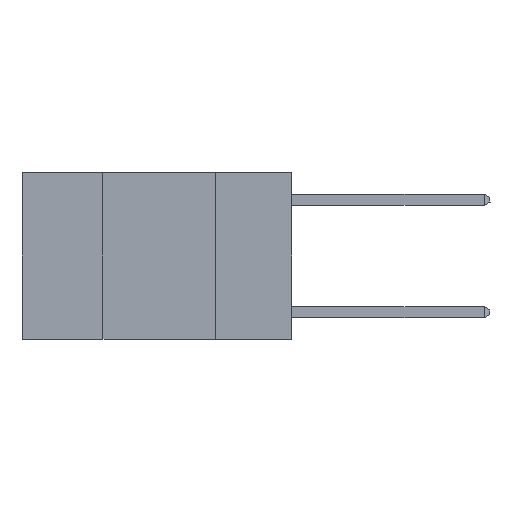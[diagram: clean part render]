
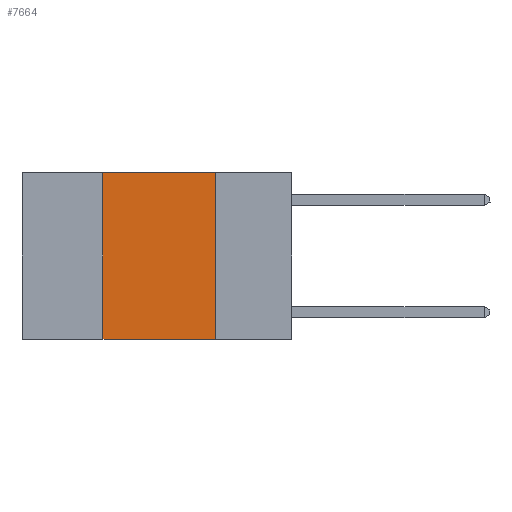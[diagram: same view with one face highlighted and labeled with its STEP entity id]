
A CAD part, left-side view. The second image highlights one B-rep face of the part: STEP entity #7664.
In plain terms, the highlighted planar face has unit normal (-1, 0, 0).
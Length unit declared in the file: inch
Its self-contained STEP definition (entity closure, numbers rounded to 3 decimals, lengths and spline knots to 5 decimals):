
#129 = DIRECTION ( 'NONE',  ( 0., -1., 0. ) ) ;
#972 = LINE ( 'NONE', #12079, #3948 ) ;
#1738 = CARTESIAN_POINT ( 'NONE',  ( 0., 0.42, -0.37 ) ) ;
#3015 = VERTEX_POINT ( 'NONE', #12639 ) ;
#3093 = VERTEX_POINT ( 'NONE', #12738 ) ;
#3166 = CARTESIAN_POINT ( 'NONE',  ( 0., 0.6, 0. ) ) ;
#3948 = VECTOR ( 'NONE', #4533, 39.37008 ) ;
#4533 = DIRECTION ( 'NONE',  ( 0., -1., 0. ) ) ;
#4829 = VERTEX_POINT ( 'NONE', #10952 ) ;
#6002 = EDGE_CURVE ( 'NONE', #7561, #3015, #972, .T. ) ;
#6048 = VECTOR ( 'NONE', #7433, 39.37008 ) ;
#6282 = FACE_OUTER_BOUND ( 'NONE', #12520, .T. ) ;
#6492 = CARTESIAN_POINT ( 'NONE',  ( 0., 0.6, 0. ) ) ;
#6706 = EDGE_CURVE ( 'NONE', #3093, #4829, #13744, .T. ) ;
#7067 = DIRECTION ( 'NONE',  ( 1., 0., 0. ) ) ;
#7218 = LINE ( 'NONE', #8104, #13854 ) ;
#7433 = DIRECTION ( 'NONE',  ( 0., 0., 1. ) ) ;
#7561 = VERTEX_POINT ( 'NONE', #1738 ) ;
#7664 = ADVANCED_FACE ( 'NONE', ( #6282 ), #14537, .F. ) ;
#8104 = CARTESIAN_POINT ( 'NONE',  ( 0., 0.17, 0. ) ) ;
#9860 = EDGE_CURVE ( 'NONE', #4829, #3015, #7218, .T. ) ;
#9919 = ORIENTED_EDGE ( 'NONE', *, *, #9860, .F. ) ;
#10024 = VECTOR ( 'NONE', #129, 39.37008 ) ;
#10835 = ORIENTED_EDGE ( 'NONE', *, *, #6706, .F. ) ;
#10885 = ORIENTED_EDGE ( 'NONE', *, *, #14345, .F. ) ;
#10952 = CARTESIAN_POINT ( 'NONE',  ( 0., 0.17, 0. ) ) ;
#11169 = ORIENTED_EDGE ( 'NONE', *, *, #6002, .T. ) ;
#12079 = CARTESIAN_POINT ( 'NONE',  ( 0., 0.6, -0.37 ) ) ;
#12520 = EDGE_LOOP ( 'NONE', ( #9919, #10835, #10885, #11169 ) ) ;
#12639 = CARTESIAN_POINT ( 'NONE',  ( 0., 0.17, -0.37 ) ) ;
#12738 = CARTESIAN_POINT ( 'NONE',  ( 0., 0.42, 0. ) ) ;
#13744 = LINE ( 'NONE', #6492, #10024 ) ;
#13854 = VECTOR ( 'NONE', #15568, 39.37008 ) ;
#14039 = AXIS2_PLACEMENT_3D ( 'NONE', #3166, #7067, #15801 ) ;
#14345 = EDGE_CURVE ( 'NONE', #7561, #3093, #16013, .T. ) ;
#14537 = PLANE ( 'NONE',  #14039 ) ;
#14908 = CARTESIAN_POINT ( 'NONE',  ( 0., 0.42, 0. ) ) ;
#15568 = DIRECTION ( 'NONE',  ( 0., 0., -1. ) ) ;
#15801 = DIRECTION ( 'NONE',  ( 0., 0., -1. ) ) ;
#16013 = LINE ( 'NONE', #14908, #6048 ) ;
